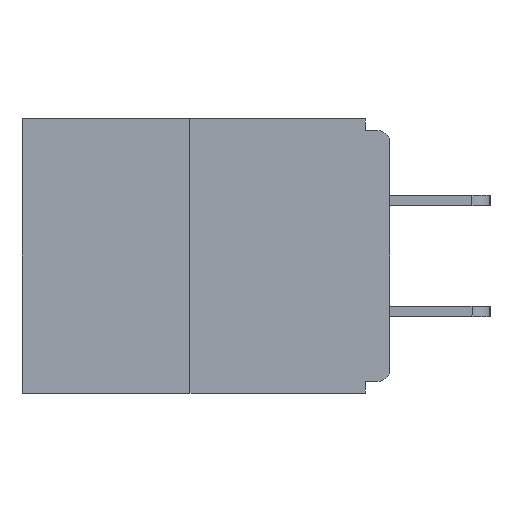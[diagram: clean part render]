
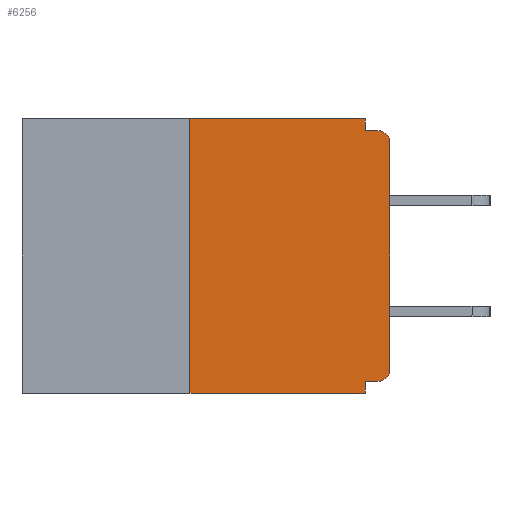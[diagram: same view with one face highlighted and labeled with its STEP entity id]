
A CAD part, left-side view. The second image highlights one B-rep face of the part: STEP entity #6256.
In plain terms, the highlighted planar face has unit normal (-1, 0, 0).
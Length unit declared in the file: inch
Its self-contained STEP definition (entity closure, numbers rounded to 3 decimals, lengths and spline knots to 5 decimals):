
#240 = DIRECTION ( 'NONE',  ( 1., 0., 0. ) ) ;
#267 = VERTEX_POINT ( 'NONE', #17230 ) ;
#369 = CARTESIAN_POINT ( 'NONE',  ( 0., 0.031, 0. ) ) ;
#575 = CARTESIAN_POINT ( 'NONE',  ( 0., 0.031, -0.328 ) ) ;
#643 = VERTEX_POINT ( 'NONE', #8722 ) ;
#705 = DIRECTION ( 'NONE',  ( -1., 0., 0. ) ) ;
#758 = CARTESIAN_POINT ( 'NONE',  ( 0., 0., 0. ) ) ;
#1753 = CARTESIAN_POINT ( 'NONE',  ( 0., 0.031, 0. ) ) ;
#2914 = DIRECTION ( 'NONE',  ( -1., 0., 0. ) ) ;
#3051 = ORIENTED_EDGE ( 'NONE', *, *, #20838, .F. ) ;
#3503 = VECTOR ( 'NONE', #5720, 39.37008 ) ;
#3788 = ORIENTED_EDGE ( 'NONE', *, *, #22687, .T. ) ;
#3839 = VERTEX_POINT ( 'NONE', #369 ) ;
#4854 = CIRCLE ( 'NONE', #20762, 0.015 ) ;
#5182 = DIRECTION ( 'NONE',  ( 0., -1., 0. ) ) ;
#5388 = VERTEX_POINT ( 'NONE', #11200 ) ;
#5453 = CARTESIAN_POINT ( 'NONE',  ( 0., 0.46, -0.343 ) ) ;
#5466 = EDGE_LOOP ( 'NONE', ( #16367, #10014, #21950, #3051, #16416, #25924, #3788, #11950, #23663, #8406 ) ) ;
#5720 = DIRECTION ( 'NONE',  ( 0., 1., 0. ) ) ;
#5786 = EDGE_CURVE ( 'NONE', #7058, #5388, #9000, .T. ) ;
#6256 = ADVANCED_FACE ( 'NONE', ( #21025 ), #8694, .F. ) ;
#6722 = LINE ( 'NONE', #24232, #26971 ) ;
#6822 = CARTESIAN_POINT ( 'NONE',  ( 0., 0.015, -0.328 ) ) ;
#7058 = VERTEX_POINT ( 'NONE', #23005 ) ;
#7564 = VECTOR ( 'NONE', #11987, 39.37008 ) ;
#8406 = ORIENTED_EDGE ( 'NONE', *, *, #12469, .F. ) ;
#8694 = PLANE ( 'NONE',  #10104 ) ;
#8722 = CARTESIAN_POINT ( 'NONE',  ( 0., 0., -0.313 ) ) ;
#9000 = LINE ( 'NONE', #21001, #22586 ) ;
#9210 = VERTEX_POINT ( 'NONE', #6822 ) ;
#9802 = CARTESIAN_POINT ( 'NONE',  ( 0., 0., -0.328 ) ) ;
#9809 = AXIS2_PLACEMENT_3D ( 'NONE', #17728, #2914, #11655 ) ;
#9873 = LINE ( 'NONE', #27009, #7564 ) ;
#10014 = ORIENTED_EDGE ( 'NONE', *, *, #5786, .F. ) ;
#10104 = AXIS2_PLACEMENT_3D ( 'NONE', #23535, #240, #15110 ) ;
#10108 = VECTOR ( 'NONE', #11447, 39.37008 ) ;
#10638 = VERTEX_POINT ( 'NONE', #575 ) ;
#10793 = LINE ( 'NONE', #19994, #10108 ) ;
#11142 = CARTESIAN_POINT ( 'NONE',  ( 0., 0.031, -0.343 ) ) ;
#11200 = CARTESIAN_POINT ( 'NONE',  ( 0., 0.25, 0. ) ) ;
#11447 = DIRECTION ( 'NONE',  ( 0., -1., 0. ) ) ;
#11655 = DIRECTION ( 'NONE',  ( 0., 0., -1. ) ) ;
#11950 = ORIENTED_EDGE ( 'NONE', *, *, #26426, .T. ) ;
#11987 = DIRECTION ( 'NONE',  ( 0., -1., 0. ) ) ;
#12469 = EDGE_CURVE ( 'NONE', #3839, #18977, #20206, .T. ) ;
#13084 = EDGE_CURVE ( 'NONE', #5388, #3839, #9873, .T. ) ;
#13263 = DIRECTION ( 'NONE',  ( 0., 0., -1. ) ) ;
#13280 = VERTEX_POINT ( 'NONE', #22333 ) ;
#14359 = EDGE_CURVE ( 'NONE', #9210, #10638, #25412, .T. ) ;
#14892 = DIRECTION ( 'NONE',  ( 0., 0., 1. ) ) ;
#15110 = DIRECTION ( 'NONE',  ( 0., 0., -1. ) ) ;
#15929 = VECTOR ( 'NONE', #16548, 39.37008 ) ;
#16211 = LINE ( 'NONE', #5453, #20473 ) ;
#16367 = ORIENTED_EDGE ( 'NONE', *, *, #13084, .F. ) ;
#16416 = ORIENTED_EDGE ( 'NONE', *, *, #14359, .F. ) ;
#16548 = DIRECTION ( 'NONE',  ( 0., 0., -1. ) ) ;
#17230 = CARTESIAN_POINT ( 'NONE',  ( 0., 0., -0.03 ) ) ;
#17610 = DIRECTION ( 'NONE',  ( 0., 0., -1. ) ) ;
#17651 = CARTESIAN_POINT ( 'NONE',  ( 0., 0.015, -0.03 ) ) ;
#17728 = CARTESIAN_POINT ( 'NONE',  ( 0., 0.015, -0.313 ) ) ;
#18875 = EDGE_CURVE ( 'NONE', #9210, #643, #21107, .T. ) ;
#18936 = VECTOR ( 'NONE', #21463, 39.37008 ) ;
#18977 = VERTEX_POINT ( 'NONE', #20274 ) ;
#19393 = VERTEX_POINT ( 'NONE', #11142 ) ;
#19994 = CARTESIAN_POINT ( 'NONE',  ( 0., 0., -0.015 ) ) ;
#20206 = LINE ( 'NONE', #1753, #15929 ) ;
#20274 = CARTESIAN_POINT ( 'NONE',  ( 0., 0.031, -0.015 ) ) ;
#20473 = VECTOR ( 'NONE', #5182, 39.37008 ) ;
#20762 = AXIS2_PLACEMENT_3D ( 'NONE', #17651, #705, #13263 ) ;
#20838 = EDGE_CURVE ( 'NONE', #10638, #19393, #6722, .T. ) ;
#21001 = CARTESIAN_POINT ( 'NONE',  ( 0., 0.25, 0. ) ) ;
#21025 = FACE_OUTER_BOUND ( 'NONE', #5466, .T. ) ;
#21107 = CIRCLE ( 'NONE', #9809, 0.015 ) ;
#21463 = DIRECTION ( 'NONE',  ( 0., 0., 1. ) ) ;
#21950 = ORIENTED_EDGE ( 'NONE', *, *, #25583, .T. ) ;
#22201 = LINE ( 'NONE', #758, #18936 ) ;
#22333 = CARTESIAN_POINT ( 'NONE',  ( 0., 0.015, -0.015 ) ) ;
#22586 = VECTOR ( 'NONE', #14892, 39.37008 ) ;
#22687 = EDGE_CURVE ( 'NONE', #643, #267, #22201, .T. ) ;
#23005 = CARTESIAN_POINT ( 'NONE',  ( 0., 0.25, -0.343 ) ) ;
#23535 = CARTESIAN_POINT ( 'NONE',  ( 0., 0.46, 0. ) ) ;
#23663 = ORIENTED_EDGE ( 'NONE', *, *, #27111, .F. ) ;
#24232 = CARTESIAN_POINT ( 'NONE',  ( 0., 0.031, -0.343 ) ) ;
#25412 = LINE ( 'NONE', #9802, #3503 ) ;
#25583 = EDGE_CURVE ( 'NONE', #7058, #19393, #16211, .T. ) ;
#25924 = ORIENTED_EDGE ( 'NONE', *, *, #18875, .T. ) ;
#26426 = EDGE_CURVE ( 'NONE', #267, #13280, #4854, .T. ) ;
#26971 = VECTOR ( 'NONE', #17610, 39.37008 ) ;
#27009 = CARTESIAN_POINT ( 'NONE',  ( 0., 0.46, 0. ) ) ;
#27111 = EDGE_CURVE ( 'NONE', #18977, #13280, #10793, .T. ) ;
